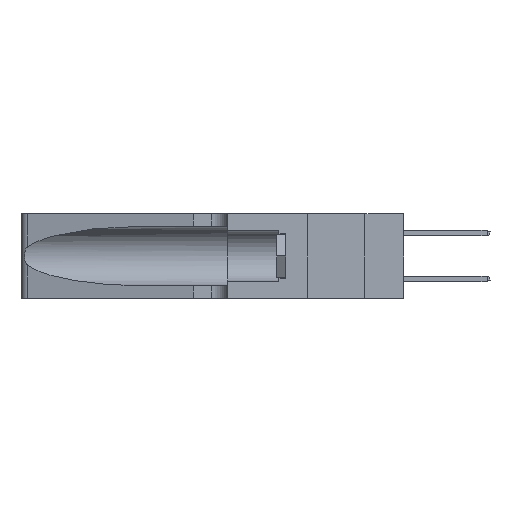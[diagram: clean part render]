
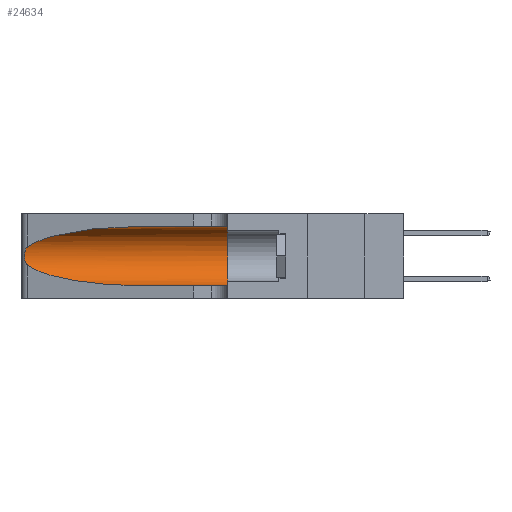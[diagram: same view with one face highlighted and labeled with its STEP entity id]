
A CAD part, left-side view. The second image highlights one B-rep face of the part: STEP entity #24634.
In plain terms, the highlighted cylindrical face has radius 3.308 mm (diameter 6.617 mm), a partial arc.
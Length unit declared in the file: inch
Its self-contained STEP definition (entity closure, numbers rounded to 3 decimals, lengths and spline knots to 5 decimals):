
#930 = ORIENTED_EDGE ( 'NONE', *, *, #21415, .F. ) ;
#1627 = AXIS2_PLACEMENT_3D ( 'NONE', #12602, #22484, #29034 ) ;
#1639 = CARTESIAN_POINT ( 'NONE',  ( 0.26018, 1.23835, 0.19895 ) ) ;
#4895 = CARTESIAN_POINT ( 'NONE',  ( 0.1305, 1.61858, 0.31525 ) ) ;
#4940 = CARTESIAN_POINT ( 'NONE',  ( 0.25555, 1.22993, 0.14849 ) ) ;
#5230 = CARTESIAN_POINT ( 'NONE',  ( 0.26017, 1.23833, 0.17102 ) ) ;
#5520 = CARTESIAN_POINT ( 'NONE',  ( 0.25487, 1.22718, 0.22369 ) ) ;
#5693 = VERTEX_POINT ( 'NONE', #38401 ) ;
#6098 = VECTOR ( 'NONE', #14643, 39.37008 ) ;
#6613 = CARTESIAN_POINT ( 'NONE',  ( 0.1305, 0.35, 0.31525 ) ) ;
#8423 = FACE_OUTER_BOUND ( 'NONE', #35947, .T. ) ;
#8500 = CARTESIAN_POINT ( 'NONE',  ( 0.2373, 1.15595, 0.08982 ) ) ;
#9866 = CARTESIAN_POINT ( 'NONE',  ( 0.1305, 0.72297, 0.31525 ) ) ;
#10723 = VERTEX_POINT ( 'NONE', #22235 ) ;
#11715 = CIRCLE ( 'NONE', #16963, 0.13025 ) ;
#11863 = CARTESIAN_POINT ( 'NONE',  ( 0.26075, 1.23896, 0.178 ) ) ;
#12147 = CARTESIAN_POINT ( 'NONE',  ( 0.26075, 1.23896, 0.19203 ) ) ;
#12240 = CARTESIAN_POINT ( 'NONE',  ( 0.18966, 0.96281, 0.31525 ) ) ;
#12602 = CARTESIAN_POINT ( 'NONE',  ( 0.1305, 1.61858, 0.185 ) ) ;
#12877 = EDGE_CURVE ( 'NONE', #34947, #32003, #34220, .T. ) ;
#14413 = LINE ( 'NONE', #4895, #40019 ) ;
#14643 = DIRECTION ( 'NONE',  ( 0., -1., 0. ) ) ;
#14883 = ORIENTED_EDGE ( 'NONE', *, *, #23022, .F. ) ;
#15045 = CARTESIAN_POINT ( 'NONE',  ( 0.25487, 1.22718, 0.14631 ) ) ;
#16963 = AXIS2_PLACEMENT_3D ( 'NONE', #37594, #18855, #38736 ) ;
#18024 = CARTESIAN_POINT ( 'NONE',  ( 0.25639, 1.23184, 0.21858 ) ) ;
#18855 = DIRECTION ( 'NONE',  ( 0., 1., 0. ) ) ;
#18906 = VERTEX_POINT ( 'NONE', #37145 ) ;
#20261 = ORIENTED_EDGE ( 'NONE', *, *, #23942, .T. ) ;
#21415 = EDGE_CURVE ( 'NONE', #34947, #30421, #14413, .T. ) ;
#22235 = CARTESIAN_POINT ( 'NONE',  ( 0.1305, 0.35, 0.05475 ) ) ;
#22484 = DIRECTION ( 'NONE',  ( 0., -1., 0. ) ) ;
#23022 = EDGE_CURVE ( 'NONE', #30421, #10723, #11715, .T. ) ;
#23942 = EDGE_CURVE ( 'NONE', #32003, #18906, #31063, .T. ) ;
#24610 = CARTESIAN_POINT ( 'NONE',  ( 0.25639, 1.23186, 0.15144 ) ) ;
#24634 = ADVANCED_FACE ( 'NONE', ( #8423 ), #32072, .F. ) ;
#25139 = CARTESIAN_POINT ( 'NONE',  ( 0.2373, 1.15595, 0.28018 ) ) ;
#26287 = CARTESIAN_POINT ( 'NONE',  ( 0.25487, 1.22718, 0.22369 ) ) ;
#26597 = LINE ( 'NONE', #37822, #6098 ) ;
#28012 = CARTESIAN_POINT ( 'NONE',  ( 0.18966, 0.96281, 0.05475 ) ) ;
#28162 = CARTESIAN_POINT ( 'NONE',  ( 0.25555, 1.22994, 0.2215 ) ) ;
#28259 = CARTESIAN_POINT ( 'NONE',  ( 0.1305, 0.72297, 0.31525 ) ) ;
#29034 = DIRECTION ( 'NONE',  ( 0., 0., -1. ) ) ;
#30421 = VERTEX_POINT ( 'NONE', #6613 ) ;
#31063 = B_SPLINE_CURVE_WITH_KNOTS ( 'NONE', 3,
 ( #5520, #28162, #18024, #41370, #38216, #1639, #12147, #11863, #5230, #35060, #37628, #24610, #4940, #15045 ),
 .UNSPECIFIED., .F., .F.,
 ( 4, 2, 2, 2, 2, 2, 4 ),
 ( 0., 0.00027, 0.00053, 0.00107, 0.0016, 0.00187, 0.00214 ),
 .UNSPECIFIED. ) ;
#31469 = CARTESIAN_POINT ( 'NONE',  ( 0.1305, 0.72297, 0.05475 ) ) ;
#32003 = VERTEX_POINT ( 'NONE', #26287 ) ;
#32072 = CYLINDRICAL_SURFACE ( 'NONE', #1627, 0.13025 ) ;
#33287 = EDGE_CURVE ( 'NONE', #5693, #10723, #26597, .T. ) ;
#34220 =( BOUNDED_CURVE ( )  B_SPLINE_CURVE ( 3, ( #28259, #12240, #25139, #38438 ),
 .UNSPECIFIED., .F., .F. ) 
 B_SPLINE_CURVE_WITH_KNOTS ( ( 4, 4 ),
 ( 1.5708, 2.84003 ),
 .UNSPECIFIED. ) 
 CURVE ( )  GEOMETRIC_REPRESENTATION_ITEM ( )  RATIONAL_B_SPLINE_CURVE ( ( 1., 0.87, 0.87, 1. ) ) 
 REPRESENTATION_ITEM ( '' )  );
#34726 = DIRECTION ( 'NONE',  ( 0., -1., 0. ) ) ;
#34947 = VERTEX_POINT ( 'NONE', #9866 ) ;
#35060 = CARTESIAN_POINT ( 'NONE',  ( 0.25856, 1.23593, 0.16098 ) ) ;
#35859 = ORIENTED_EDGE ( 'NONE', *, *, #12877, .T. ) ;
#35947 = EDGE_LOOP ( 'NONE', ( #35859, #20261, #40949, #39839, #14883, #930 ) ) ;
#37145 = CARTESIAN_POINT ( 'NONE',  ( 0.25487, 1.22718, 0.14631 ) ) ;
#37442 = EDGE_CURVE ( 'NONE', #18906, #5693, #40794, .T. ) ;
#37594 = CARTESIAN_POINT ( 'NONE',  ( 0.1305, 0.35, 0.185 ) ) ;
#37628 = CARTESIAN_POINT ( 'NONE',  ( 0.25789, 1.23486, 0.15765 ) ) ;
#37822 = CARTESIAN_POINT ( 'NONE',  ( 0.1305, 1.61858, 0.05475 ) ) ;
#38216 = CARTESIAN_POINT ( 'NONE',  ( 0.25854, 1.2359, 0.20912 ) ) ;
#38401 = CARTESIAN_POINT ( 'NONE',  ( 0.1305, 0.72297, 0.05475 ) ) ;
#38438 = CARTESIAN_POINT ( 'NONE',  ( 0.25487, 1.22718, 0.22369 ) ) ;
#38465 = CARTESIAN_POINT ( 'NONE',  ( 0.25487, 1.22718, 0.14631 ) ) ;
#38736 = DIRECTION ( 'NONE',  ( 0., 0., 1. ) ) ;
#39839 = ORIENTED_EDGE ( 'NONE', *, *, #33287, .T. ) ;
#40019 = VECTOR ( 'NONE', #34726, 39.37008 ) ;
#40794 =( BOUNDED_CURVE ( )  B_SPLINE_CURVE ( 3, ( #38465, #8500, #28012, #31469 ),
 .UNSPECIFIED., .F., .F. ) 
 B_SPLINE_CURVE_WITH_KNOTS ( ( 4, 4 ),
 ( 3.44316, 4.71239 ),
 .UNSPECIFIED. ) 
 CURVE ( )  GEOMETRIC_REPRESENTATION_ITEM ( )  RATIONAL_B_SPLINE_CURVE ( ( 1., 0.87, 0.87, 1. ) ) 
 REPRESENTATION_ITEM ( '' )  );
#40949 = ORIENTED_EDGE ( 'NONE', *, *, #37442, .T. ) ;
#41370 = CARTESIAN_POINT ( 'NONE',  ( 0.25787, 1.23484, 0.2124 ) ) ;
